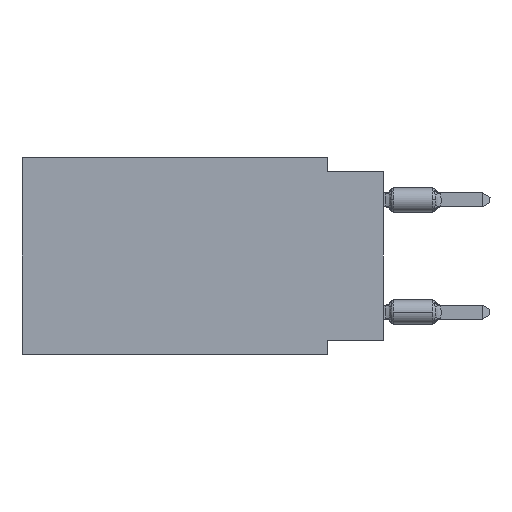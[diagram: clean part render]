
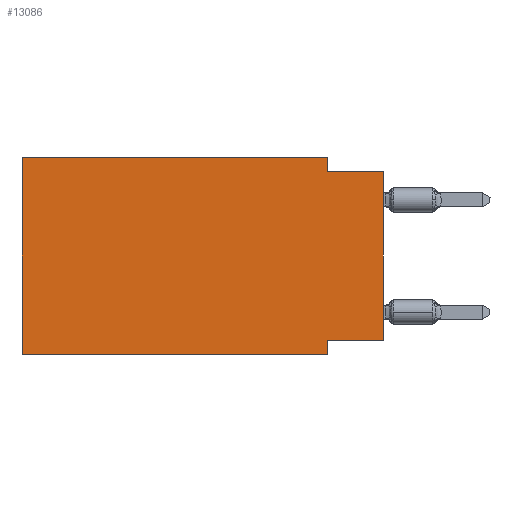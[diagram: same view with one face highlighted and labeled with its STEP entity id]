
A CAD part, left-side view. The second image highlights one B-rep face of the part: STEP entity #13086.
In plain terms, the highlighted planar face has unit normal (-1, 0, 0).
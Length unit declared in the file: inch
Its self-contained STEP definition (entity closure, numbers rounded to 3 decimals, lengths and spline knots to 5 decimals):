
#34 = PLANE ( 'NONE',  #37464 ) ;
#237 = CARTESIAN_POINT ( 'NONE',  ( 0., 0.645, 0. ) ) ;
#357 = CARTESIAN_POINT ( 'NONE',  ( 0., 0.645, 0. ) ) ;
#1093 = VERTEX_POINT ( 'NONE', #30307 ) ;
#1323 = VECTOR ( 'NONE', #17807, 39.37008 ) ;
#2073 = VECTOR ( 'NONE', #38055, 39.37008 ) ;
#2313 = ORIENTED_EDGE ( 'NONE', *, *, #40136, .F. ) ;
#2516 = CARTESIAN_POINT ( 'NONE',  ( 0., 0., -0.325 ) ) ;
#3856 = EDGE_CURVE ( 'NONE', #13210, #17334, #6404, .T. ) ;
#5094 = LINE ( 'NONE', #14930, #1323 ) ;
#5125 = DIRECTION ( 'NONE',  ( 0., 0., -1. ) ) ;
#6077 = DIRECTION ( 'NONE',  ( 0., 0., 1. ) ) ;
#6404 = LINE ( 'NONE', #28500, #31232 ) ;
#7054 = ORIENTED_EDGE ( 'NONE', *, *, #40309, .F. ) ;
#7209 = CARTESIAN_POINT ( 'NONE',  ( 0., 0.645, 0. ) ) ;
#7571 = CARTESIAN_POINT ( 'NONE',  ( 0., 0.1, -0.025 ) ) ;
#8004 = EDGE_CURVE ( 'NONE', #22416, #16351, #30486, .T. ) ;
#9091 = DIRECTION ( 'NONE',  ( 0., 0., -1. ) ) ;
#11193 = ORIENTED_EDGE ( 'NONE', *, *, #36077, .T. ) ;
#13086 = ADVANCED_FACE ( 'NONE', ( #36917 ), #34, .F. ) ;
#13096 = LINE ( 'NONE', #357, #2073 ) ;
#13210 = VERTEX_POINT ( 'NONE', #26049 ) ;
#13214 = DIRECTION ( 'NONE',  ( 0., -1., 0. ) ) ;
#14930 = CARTESIAN_POINT ( 'NONE',  ( 0., 0.645, -0.35 ) ) ;
#15654 = DIRECTION ( 'NONE',  ( 0., 0., 1. ) ) ;
#15738 = LINE ( 'NONE', #40297, #25464 ) ;
#16351 = VERTEX_POINT ( 'NONE', #20439 ) ;
#17199 = ORIENTED_EDGE ( 'NONE', *, *, #35936, .T. ) ;
#17334 = VERTEX_POINT ( 'NONE', #7209 ) ;
#17807 = DIRECTION ( 'NONE',  ( 0., -1., 0. ) ) ;
#18176 = ORIENTED_EDGE ( 'NONE', *, *, #29778, .F. ) ;
#18251 = CARTESIAN_POINT ( 'NONE',  ( 0., 0.1, 0. ) ) ;
#20439 = CARTESIAN_POINT ( 'NONE',  ( 0., 0.1, -0.35 ) ) ;
#20984 = CARTESIAN_POINT ( 'NONE',  ( 0., 0.1, -0.325 ) ) ;
#21199 = CARTESIAN_POINT ( 'NONE',  ( 0., 0.1, 0. ) ) ;
#21338 = LINE ( 'NONE', #2516, #35974 ) ;
#22416 = VERTEX_POINT ( 'NONE', #20984 ) ;
#22468 = ORIENTED_EDGE ( 'NONE', *, *, #38126, .F. ) ;
#22511 = EDGE_LOOP ( 'NONE', ( #11193, #7054, #2313, #22468, #25552, #17199, #33492, #18176 ) ) ;
#25464 = VECTOR ( 'NONE', #6077, 39.37008 ) ;
#25552 = ORIENTED_EDGE ( 'NONE', *, *, #3856, .F. ) ;
#26049 = CARTESIAN_POINT ( 'NONE',  ( 0., 0.645, -0.35 ) ) ;
#27119 = DIRECTION ( 'NONE',  ( 0., 0., -1. ) ) ;
#28314 = VERTEX_POINT ( 'NONE', #18251 ) ;
#28500 = CARTESIAN_POINT ( 'NONE',  ( 0., 0.645, 0. ) ) ;
#28955 = LINE ( 'NONE', #35502, #34990 ) ;
#29778 = EDGE_CURVE ( 'NONE', #40127, #22416, #21338, .T. ) ;
#30307 = CARTESIAN_POINT ( 'NONE',  ( 0., 0., -0.025 ) ) ;
#30486 = LINE ( 'NONE', #33166, #30487 ) ;
#30487 = VECTOR ( 'NONE', #5125, 39.37008 ) ;
#31232 = VECTOR ( 'NONE', #15654, 39.37008 ) ;
#33166 = CARTESIAN_POINT ( 'NONE',  ( 0., 0.1, -0.35 ) ) ;
#33472 = LINE ( 'NONE', #21199, #35669 ) ;
#33492 = ORIENTED_EDGE ( 'NONE', *, *, #8004, .F. ) ;
#33944 = VERTEX_POINT ( 'NONE', #7571 ) ;
#34205 = DIRECTION ( 'NONE',  ( 0., 1., 0. ) ) ;
#34990 = VECTOR ( 'NONE', #13214, 39.37008 ) ;
#35502 = CARTESIAN_POINT ( 'NONE',  ( 0., 0., -0.025 ) ) ;
#35669 = VECTOR ( 'NONE', #27119, 39.37008 ) ;
#35936 = EDGE_CURVE ( 'NONE', #13210, #16351, #5094, .T. ) ;
#35974 = VECTOR ( 'NONE', #34205, 39.37008 ) ;
#36077 = EDGE_CURVE ( 'NONE', #40127, #1093, #15738, .T. ) ;
#36917 = FACE_OUTER_BOUND ( 'NONE', #22511, .T. ) ;
#37464 = AXIS2_PLACEMENT_3D ( 'NONE', #237, #37518, #9091 ) ;
#37518 = DIRECTION ( 'NONE',  ( 1., 0., 0. ) ) ;
#38055 = DIRECTION ( 'NONE',  ( 0., -1., 0. ) ) ;
#38126 = EDGE_CURVE ( 'NONE', #17334, #28314, #13096, .T. ) ;
#39627 = CARTESIAN_POINT ( 'NONE',  ( 0., 0., -0.325 ) ) ;
#40127 = VERTEX_POINT ( 'NONE', #39627 ) ;
#40136 = EDGE_CURVE ( 'NONE', #28314, #33944, #33472, .T. ) ;
#40297 = CARTESIAN_POINT ( 'NONE',  ( 0., 0., 0. ) ) ;
#40309 = EDGE_CURVE ( 'NONE', #33944, #1093, #28955, .T. ) ;
